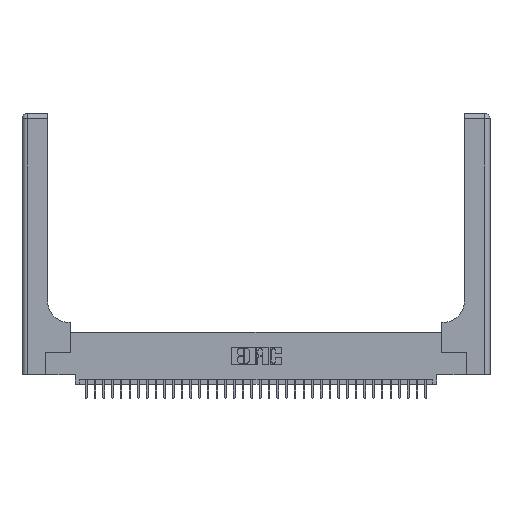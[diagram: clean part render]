
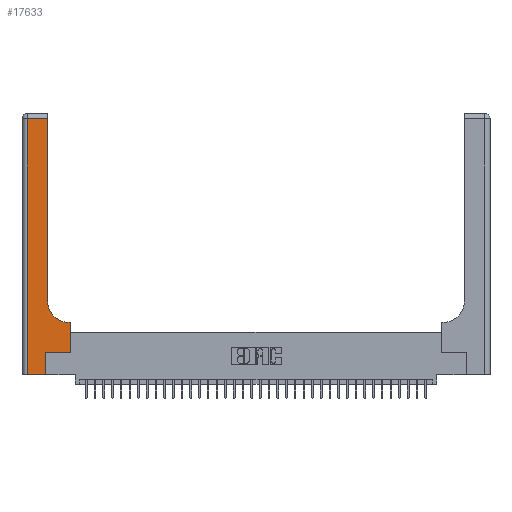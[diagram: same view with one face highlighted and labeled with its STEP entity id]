
A CAD part, top view. The second image highlights one B-rep face of the part: STEP entity #17633.
In plain terms, the highlighted planar face has unit normal (0, 0, 1).
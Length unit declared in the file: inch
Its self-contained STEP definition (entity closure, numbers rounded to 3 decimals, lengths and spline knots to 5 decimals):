
#264 = EDGE_CURVE ( 'NONE', #25777, #23431, #14706, .T. ) ;
#407 = CARTESIAN_POINT ( 'NONE',  ( 0.269, 0.25, 0.37 ) ) ;
#1020 = CARTESIAN_POINT ( 'NONE',  ( 0.06, 2.94, 0.37 ) ) ;
#1653 = ORIENTED_EDGE ( 'NONE', *, *, #32703, .T. ) ;
#1844 = DIRECTION ( 'NONE',  ( 0., 1., 0. ) ) ;
#2499 = VECTOR ( 'NONE', #31095, 39.37008 ) ;
#2553 = DIRECTION ( 'NONE',  ( 1., 0., 0. ) ) ;
#2574 = ORIENTED_EDGE ( 'NONE', *, *, #16324, .T. ) ;
#2971 = AXIS2_PLACEMENT_3D ( 'NONE', #25020, #7785, #27849 ) ;
#3482 = ORIENTED_EDGE ( 'NONE', *, *, #264, .T. ) ;
#3648 = EDGE_CURVE ( 'NONE', #19965, #18453, #25547, .T. ) ;
#3762 = VERTEX_POINT ( 'NONE', #11727 ) ;
#4829 = ORIENTED_EDGE ( 'NONE', *, *, #36810, .T. ) ;
#6173 = DIRECTION ( 'NONE',  ( -1., 0., 0. ) ) ;
#7013 = CARTESIAN_POINT ( 'NONE',  ( 0.5585, 0.25, 0.37 ) ) ;
#7186 = VECTOR ( 'NONE', #25742, 39.37008 ) ;
#7785 = DIRECTION ( 'NONE',  ( 0., 0., -1. ) ) ;
#9025 = CARTESIAN_POINT ( 'NONE',  ( 0., 3., 0.37 ) ) ;
#9093 = DIRECTION ( 'NONE',  ( 0., 1., 0. ) ) ;
#11318 = LINE ( 'NONE', #13750, #18062 ) ;
#11727 = CARTESIAN_POINT ( 'NONE',  ( 0.2915, 0.85, 0.37 ) ) ;
#12173 = CARTESIAN_POINT ( 'NONE',  ( 0.06, 0., 0.37 ) ) ;
#12699 = VERTEX_POINT ( 'NONE', #407 ) ;
#12879 = VERTEX_POINT ( 'NONE', #15608 ) ;
#13750 = CARTESIAN_POINT ( 'NONE',  ( 0.2915, 3., 0.37 ) ) ;
#14706 = LINE ( 'NONE', #7013, #29786 ) ;
#15608 = CARTESIAN_POINT ( 'NONE',  ( 0.269, 0., 0.37 ) ) ;
#16324 = EDGE_CURVE ( 'NONE', #12699, #25777, #23861, .T. ) ;
#16356 = DIRECTION ( 'NONE',  ( 1., 0., 0. ) ) ;
#17024 = CARTESIAN_POINT ( 'NONE',  ( 0.5415, 0.6, 0.37 ) ) ;
#17633 = ADVANCED_FACE ( 'NONE', ( #26383 ), #20646, .F. ) ;
#17725 = CARTESIAN_POINT ( 'NONE',  ( 0.269, 0., 0.37 ) ) ;
#18062 = VECTOR ( 'NONE', #1844, 39.37008 ) ;
#18121 = AXIS2_PLACEMENT_3D ( 'NONE', #9025, #23501, #6173 ) ;
#18453 = VERTEX_POINT ( 'NONE', #1020 ) ;
#19868 = ORIENTED_EDGE ( 'NONE', *, *, #22087, .T. ) ;
#19965 = VERTEX_POINT ( 'NONE', #34940 ) ;
#19972 = CARTESIAN_POINT ( 'NONE',  ( 0., 0., 0.37 ) ) ;
#20646 = PLANE ( 'NONE',  #18121 ) ;
#20775 = VECTOR ( 'NONE', #35553, 39.37008 ) ;
#21183 = ORIENTED_EDGE ( 'NONE', *, *, #3648, .T. ) ;
#21682 = LINE ( 'NONE', #31396, #7186 ) ;
#21952 = EDGE_CURVE ( 'NONE', #23431, #33884, #33964, .T. ) ;
#22081 = ORIENTED_EDGE ( 'NONE', *, *, #31512, .T. ) ;
#22087 = EDGE_CURVE ( 'NONE', #33884, #3762, #22109, .T. ) ;
#22109 = CIRCLE ( 'NONE', #2971, 0.25 ) ;
#23431 = VERTEX_POINT ( 'NONE', #34838 ) ;
#23501 = DIRECTION ( 'NONE',  ( 0., 0., -1. ) ) ;
#23861 = LINE ( 'NONE', #33271, #24743 ) ;
#24161 = VECTOR ( 'NONE', #9093, 39.37008 ) ;
#24289 = DIRECTION ( 'NONE',  ( 0., 1., 0. ) ) ;
#24736 = ORIENTED_EDGE ( 'NONE', *, *, #32814, .T. ) ;
#24743 = VECTOR ( 'NONE', #16356, 39.37008 ) ;
#25020 = CARTESIAN_POINT ( 'NONE',  ( 0.5415, 0.85, 0.37 ) ) ;
#25547 = LINE ( 'NONE', #33893, #2499 ) ;
#25742 = DIRECTION ( 'NONE',  ( 0., -1., 0. ) ) ;
#25777 = VERTEX_POINT ( 'NONE', #28123 ) ;
#26383 = FACE_OUTER_BOUND ( 'NONE', #26722, .T. ) ;
#26476 = ORIENTED_EDGE ( 'NONE', *, *, #21952, .T. ) ;
#26722 = EDGE_LOOP ( 'NONE', ( #4829, #21183, #22081, #1653, #24736, #2574, #3482, #26476, #19868 ) ) ;
#27849 = DIRECTION ( 'NONE',  ( 1., 0., 0. ) ) ;
#27895 = VERTEX_POINT ( 'NONE', #12173 ) ;
#28123 = CARTESIAN_POINT ( 'NONE',  ( 0.5585, 0.25, 0.37 ) ) ;
#28949 = VECTOR ( 'NONE', #2553, 39.37008 ) ;
#29786 = VECTOR ( 'NONE', #24289, 39.37008 ) ;
#30050 = CARTESIAN_POINT ( 'NONE',  ( 0.2915, 0.6, 0.37 ) ) ;
#31095 = DIRECTION ( 'NONE',  ( -1., 0., 0. ) ) ;
#31396 = CARTESIAN_POINT ( 'NONE',  ( 0.06, 3., 0.37 ) ) ;
#31512 = EDGE_CURVE ( 'NONE', #18453, #27895, #21682, .T. ) ;
#32000 = LINE ( 'NONE', #17725, #24161 ) ;
#32703 = EDGE_CURVE ( 'NONE', #27895, #12879, #35489, .T. ) ;
#32814 = EDGE_CURVE ( 'NONE', #12879, #12699, #32000, .T. ) ;
#33271 = CARTESIAN_POINT ( 'NONE',  ( 0.269, 0.25, 0.37 ) ) ;
#33884 = VERTEX_POINT ( 'NONE', #17024 ) ;
#33893 = CARTESIAN_POINT ( 'NONE',  ( 0., 2.94, 0.37 ) ) ;
#33964 = LINE ( 'NONE', #30050, #20775 ) ;
#34838 = CARTESIAN_POINT ( 'NONE',  ( 0.5585, 0.6, 0.37 ) ) ;
#34940 = CARTESIAN_POINT ( 'NONE',  ( 0.2915, 2.94, 0.37 ) ) ;
#35489 = LINE ( 'NONE', #19972, #28949 ) ;
#35553 = DIRECTION ( 'NONE',  ( -1., 0., 0. ) ) ;
#36810 = EDGE_CURVE ( 'NONE', #3762, #19965, #11318, .T. ) ;
